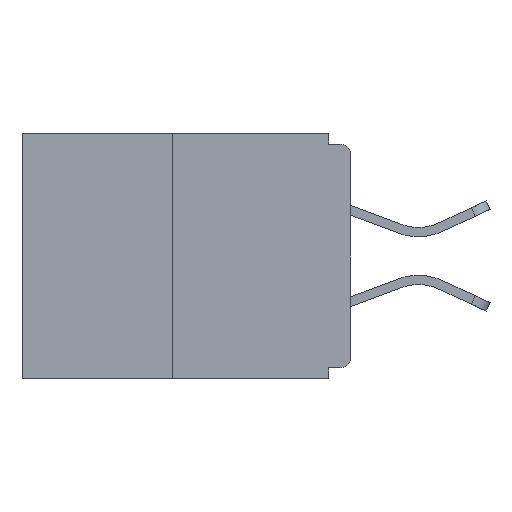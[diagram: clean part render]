
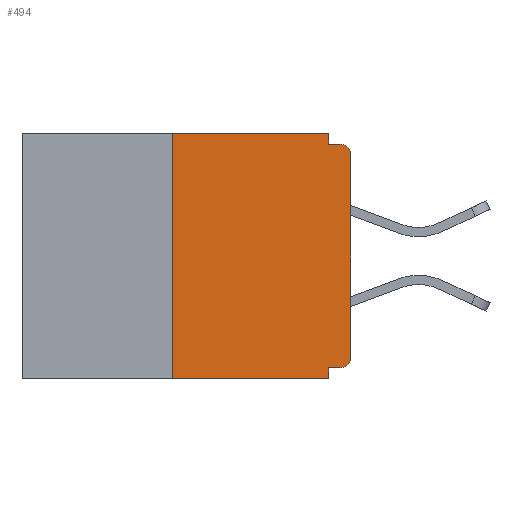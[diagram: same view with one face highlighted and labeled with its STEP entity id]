
A CAD part, left-side view. The second image highlights one B-rep face of the part: STEP entity #494.
In plain terms, the highlighted planar face has unit normal (-1, 0, 0).
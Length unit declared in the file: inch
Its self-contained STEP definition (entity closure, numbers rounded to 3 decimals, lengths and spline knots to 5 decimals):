
#61 = ORIENTED_EDGE ( 'NONE', *, *, #15344, .F. ) ;
#360 = EDGE_CURVE ( 'NONE', #4559, #7641, #13269, .T. ) ;
#422 = DIRECTION ( 'NONE',  ( 0., 0., -1. ) ) ;
#494 = ADVANCED_FACE ( 'NONE', ( #12939 ), #1861, .F. ) ;
#698 = VERTEX_POINT ( 'NONE', #13328 ) ;
#1413 = ORIENTED_EDGE ( 'NONE', *, *, #1469, .F. ) ;
#1433 = ORIENTED_EDGE ( 'NONE', *, *, #7062, .F. ) ;
#1469 = EDGE_CURVE ( 'NONE', #11899, #698, #16133, .T. ) ;
#1548 = EDGE_CURVE ( 'NONE', #5430, #26563, #12575, .T. ) ;
#1827 = CARTESIAN_POINT ( 'NONE',  ( 0., 0., 0. ) ) ;
#1861 = PLANE ( 'NONE',  #18751 ) ;
#2686 = DIRECTION ( 'NONE',  ( 0., 0., -1. ) ) ;
#2839 = CARTESIAN_POINT ( 'NONE',  ( 0., 0.25, 0. ) ) ;
#3173 = ORIENTED_EDGE ( 'NONE', *, *, #4560, .F. ) ;
#4103 = CARTESIAN_POINT ( 'NONE',  ( 0., 0.031, -0.015 ) ) ;
#4452 = CARTESIAN_POINT ( 'NONE',  ( 0., 0.031, -0.343 ) ) ;
#4559 = VERTEX_POINT ( 'NONE', #12969 ) ;
#4560 = EDGE_CURVE ( 'NONE', #19320, #26563, #5059, .T. ) ;
#4795 = CARTESIAN_POINT ( 'NONE',  ( 0., 0.25, -0.343 ) ) ;
#4835 = CARTESIAN_POINT ( 'NONE',  ( 0., 0.015, -0.03 ) ) ;
#5059 = LINE ( 'NONE', #4452, #5731 ) ;
#5430 = VERTEX_POINT ( 'NONE', #4795 ) ;
#5686 = ORIENTED_EDGE ( 'NONE', *, *, #17817, .F. ) ;
#5731 = VECTOR ( 'NONE', #25349, 39.37008 ) ;
#6156 = CIRCLE ( 'NONE', #25470, 0.015 ) ;
#7040 = VECTOR ( 'NONE', #17610, 39.37008 ) ;
#7062 = EDGE_CURVE ( 'NONE', #17003, #15167, #25728, .T. ) ;
#7641 = VERTEX_POINT ( 'NONE', #20866 ) ;
#7782 = CIRCLE ( 'NONE', #22235, 0.015 ) ;
#7847 = VECTOR ( 'NONE', #13525, 39.37008 ) ;
#7989 = CARTESIAN_POINT ( 'NONE',  ( 0., 0.46, 0. ) ) ;
#8230 = CARTESIAN_POINT ( 'NONE',  ( 0., 0.031, 0. ) ) ;
#9416 = ORIENTED_EDGE ( 'NONE', *, *, #1548, .T. ) ;
#9489 = ORIENTED_EDGE ( 'NONE', *, *, #24825, .F. ) ;
#10116 = CARTESIAN_POINT ( 'NONE',  ( 0., 0.46, 0. ) ) ;
#10646 = VECTOR ( 'NONE', #21357, 39.37008 ) ;
#10880 = DIRECTION ( 'NONE',  ( 0., 0., -1. ) ) ;
#11132 = ORIENTED_EDGE ( 'NONE', *, *, #12562, .T. ) ;
#11844 = CARTESIAN_POINT ( 'NONE',  ( 0., 0.031, -0.343 ) ) ;
#11899 = VERTEX_POINT ( 'NONE', #4103 ) ;
#12562 = EDGE_CURVE ( 'NONE', #19966, #4559, #6156, .T. ) ;
#12575 = LINE ( 'NONE', #19768, #7040 ) ;
#12939 = FACE_OUTER_BOUND ( 'NONE', #18963, .T. ) ;
#12969 = CARTESIAN_POINT ( 'NONE',  ( 0., 0., -0.313 ) ) ;
#13269 = LINE ( 'NONE', #1827, #26620 ) ;
#13328 = CARTESIAN_POINT ( 'NONE',  ( 0., 0.015, -0.015 ) ) ;
#13525 = DIRECTION ( 'NONE',  ( 0., 0., 1. ) ) ;
#13677 = VECTOR ( 'NONE', #26691, 39.37008 ) ;
#13792 = ORIENTED_EDGE ( 'NONE', *, *, #19346, .T. ) ;
#14645 = VECTOR ( 'NONE', #18250, 39.37008 ) ;
#14721 = LINE ( 'NONE', #19136, #20589 ) ;
#15167 = VERTEX_POINT ( 'NONE', #8230 ) ;
#15344 = EDGE_CURVE ( 'NONE', #15167, #11899, #14721, .T. ) ;
#16133 = LINE ( 'NONE', #17335, #10646 ) ;
#17003 = VERTEX_POINT ( 'NONE', #25440 ) ;
#17175 = DIRECTION ( 'NONE',  ( -1., 0., 0. ) ) ;
#17335 = CARTESIAN_POINT ( 'NONE',  ( 0., 0., -0.015 ) ) ;
#17610 = DIRECTION ( 'NONE',  ( 0., -1., 0. ) ) ;
#17817 = EDGE_CURVE ( 'NONE', #19966, #19320, #22132, .T. ) ;
#18250 = DIRECTION ( 'NONE',  ( 0., 1., 0. ) ) ;
#18751 = AXIS2_PLACEMENT_3D ( 'NONE', #10116, #24643, #26730 ) ;
#18963 = EDGE_LOOP ( 'NONE', ( #1433, #9489, #9416, #3173, #5686, #11132, #26190, #13792, #1413, #61 ) ) ;
#19136 = CARTESIAN_POINT ( 'NONE',  ( 0., 0.031, 0. ) ) ;
#19320 = VERTEX_POINT ( 'NONE', #26805 ) ;
#19346 = EDGE_CURVE ( 'NONE', #7641, #698, #7782, .T. ) ;
#19768 = CARTESIAN_POINT ( 'NONE',  ( 0., 0.46, -0.343 ) ) ;
#19773 = CARTESIAN_POINT ( 'NONE',  ( 0., 0., -0.328 ) ) ;
#19966 = VERTEX_POINT ( 'NONE', #22592 ) ;
#20589 = VECTOR ( 'NONE', #422, 39.37008 ) ;
#20866 = CARTESIAN_POINT ( 'NONE',  ( 0., 0., -0.03 ) ) ;
#21203 = CARTESIAN_POINT ( 'NONE',  ( 0., 0.015, -0.313 ) ) ;
#21357 = DIRECTION ( 'NONE',  ( 0., -1., 0. ) ) ;
#22132 = LINE ( 'NONE', #19773, #14645 ) ;
#22235 = AXIS2_PLACEMENT_3D ( 'NONE', #4835, #17175, #2686 ) ;
#22592 = CARTESIAN_POINT ( 'NONE',  ( 0., 0.015, -0.328 ) ) ;
#23317 = DIRECTION ( 'NONE',  ( -1., 0., 0. ) ) ;
#24643 = DIRECTION ( 'NONE',  ( 1., 0., 0. ) ) ;
#24825 = EDGE_CURVE ( 'NONE', #5430, #17003, #26008, .T. ) ;
#25266 = DIRECTION ( 'NONE',  ( 0., 0., 1. ) ) ;
#25349 = DIRECTION ( 'NONE',  ( 0., 0., -1. ) ) ;
#25440 = CARTESIAN_POINT ( 'NONE',  ( 0., 0.25, 0. ) ) ;
#25470 = AXIS2_PLACEMENT_3D ( 'NONE', #21203, #23317, #10880 ) ;
#25728 = LINE ( 'NONE', #7989, #13677 ) ;
#26008 = LINE ( 'NONE', #2839, #7847 ) ;
#26190 = ORIENTED_EDGE ( 'NONE', *, *, #360, .T. ) ;
#26563 = VERTEX_POINT ( 'NONE', #11844 ) ;
#26620 = VECTOR ( 'NONE', #25266, 39.37008 ) ;
#26691 = DIRECTION ( 'NONE',  ( 0., -1., 0. ) ) ;
#26730 = DIRECTION ( 'NONE',  ( 0., 0., -1. ) ) ;
#26805 = CARTESIAN_POINT ( 'NONE',  ( 0., 0.031, -0.328 ) ) ;
